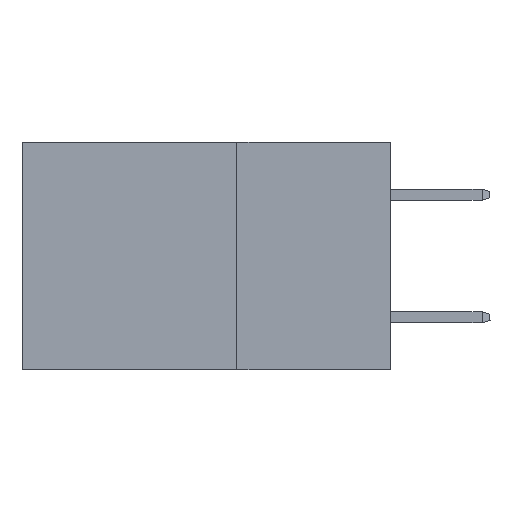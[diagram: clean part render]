
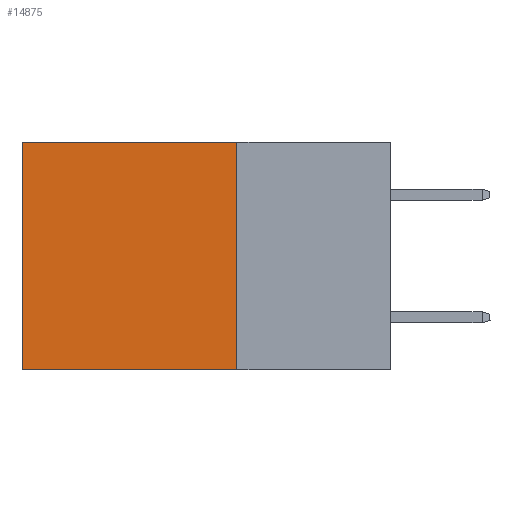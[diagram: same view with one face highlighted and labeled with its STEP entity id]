
A CAD part, left-side view. The second image highlights one B-rep face of the part: STEP entity #14875.
In plain terms, the highlighted planar face has unit normal (-1, 0, 0).
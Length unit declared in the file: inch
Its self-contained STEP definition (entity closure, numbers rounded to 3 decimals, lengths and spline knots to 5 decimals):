
#994 = ORIENTED_EDGE ( 'NONE', *, *, #24533, .F. ) ;
#1290 = CARTESIAN_POINT ( 'NONE',  ( 0.2875, 0.25, 0. ) ) ;
#1546 = LINE ( 'NONE', #19149, #6274 ) ;
#1556 = VERTEX_POINT ( 'NONE', #5541 ) ;
#3724 = VERTEX_POINT ( 'NONE', #22878 ) ;
#3791 = CARTESIAN_POINT ( 'NONE',  ( 0.2875, 0.6, 0. ) ) ;
#4293 = ORIENTED_EDGE ( 'NONE', *, *, #20429, .F. ) ;
#5541 = CARTESIAN_POINT ( 'NONE',  ( 0.2875, 0.6, 0. ) ) ;
#5689 = FACE_OUTER_BOUND ( 'NONE', #8753, .T. ) ;
#5965 = PLANE ( 'NONE',  #9254 ) ;
#6274 = VECTOR ( 'NONE', #22871, 39.37008 ) ;
#8374 = LINE ( 'NONE', #17108, #8924 ) ;
#8578 = VERTEX_POINT ( 'NONE', #20467 ) ;
#8753 = EDGE_LOOP ( 'NONE', ( #24087, #4293, #994, #17443 ) ) ;
#8924 = VECTOR ( 'NONE', #24760, 39.37008 ) ;
#9254 = AXIS2_PLACEMENT_3D ( 'NONE', #21527, #19248, #10381 ) ;
#10381 = DIRECTION ( 'NONE',  ( 0., 0., -1. ) ) ;
#12038 = LINE ( 'NONE', #1290, #14001 ) ;
#12095 = DIRECTION ( 'NONE',  ( 0., 0., -1. ) ) ;
#14001 = VECTOR ( 'NONE', #18759, 39.37008 ) ;
#14875 = ADVANCED_FACE ( 'NONE', ( #5689 ), #5965, .F. ) ;
#15269 = VERTEX_POINT ( 'NONE', #17484 ) ;
#17108 = CARTESIAN_POINT ( 'NONE',  ( 0.2875, 0.25, -0.37 ) ) ;
#17443 = ORIENTED_EDGE ( 'NONE', *, *, #21600, .T. ) ;
#17484 = CARTESIAN_POINT ( 'NONE',  ( 0.2875, 0.6, -0.37 ) ) ;
#18573 = EDGE_CURVE ( 'NONE', #1556, #15269, #18958, .T. ) ;
#18759 = DIRECTION ( 'NONE',  ( 0., 1., 0. ) ) ;
#18958 = LINE ( 'NONE', #3791, #21718 ) ;
#19149 = CARTESIAN_POINT ( 'NONE',  ( 0.2875, 0.25, 0. ) ) ;
#19248 = DIRECTION ( 'NONE',  ( 1., 0., 0. ) ) ;
#20429 = EDGE_CURVE ( 'NONE', #8578, #15269, #8374, .T. ) ;
#20467 = CARTESIAN_POINT ( 'NONE',  ( 0.2875, 0.25, -0.37 ) ) ;
#21527 = CARTESIAN_POINT ( 'NONE',  ( 0.2875, 0.25, 0. ) ) ;
#21600 = EDGE_CURVE ( 'NONE', #3724, #1556, #12038, .T. ) ;
#21718 = VECTOR ( 'NONE', #12095, 39.37008 ) ;
#22871 = DIRECTION ( 'NONE',  ( 0., 0., -1. ) ) ;
#22878 = CARTESIAN_POINT ( 'NONE',  ( 0.2875, 0.25, 0. ) ) ;
#24087 = ORIENTED_EDGE ( 'NONE', *, *, #18573, .T. ) ;
#24533 = EDGE_CURVE ( 'NONE', #3724, #8578, #1546, .T. ) ;
#24760 = DIRECTION ( 'NONE',  ( 0., 1., 0. ) ) ;
